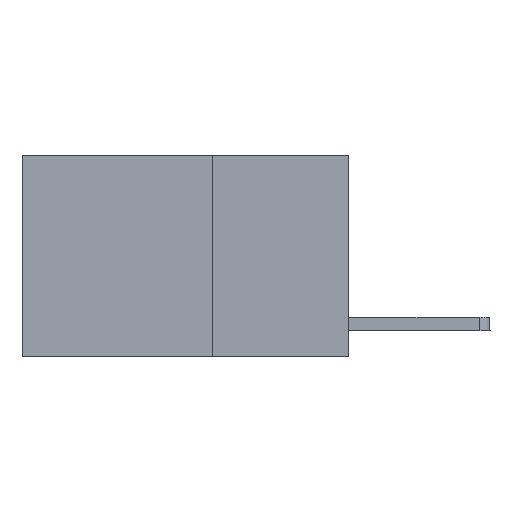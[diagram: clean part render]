
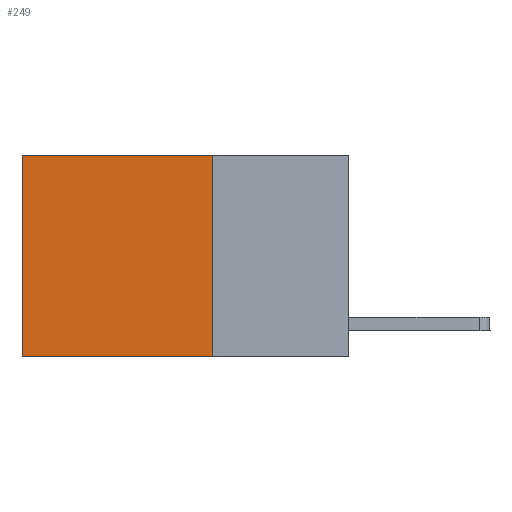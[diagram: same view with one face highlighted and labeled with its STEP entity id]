
A CAD part, left-side view. The second image highlights one B-rep face of the part: STEP entity #249.
In plain terms, the highlighted planar face has unit normal (-1, 0, 0).
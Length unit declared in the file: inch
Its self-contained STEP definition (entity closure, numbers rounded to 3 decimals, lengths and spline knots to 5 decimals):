
#249 = ADVANCED_FACE ( 'NONE', ( #1845 ), #5765, .F. ) ;
#305 = EDGE_CURVE ( 'NONE', #8486, #8757, #1118, .T. ) ;
#349 = ORIENTED_EDGE ( 'NONE', *, *, #305, .T. ) ;
#411 = LINE ( 'NONE', #3194, #6220 ) ;
#432 = EDGE_CURVE ( 'NONE', #8757, #2724, #976, .T. ) ;
#976 = LINE ( 'NONE', #3034, #7132 ) ;
#1118 = LINE ( 'NONE', #3878, #6696 ) ;
#1363 = LINE ( 'NONE', #4115, #3870 ) ;
#1447 = ORIENTED_EDGE ( 'NONE', *, *, #4941, .F. ) ;
#1714 = DIRECTION ( 'NONE',  ( 1., 0., 0. ) ) ;
#1845 = FACE_OUTER_BOUND ( 'NONE', #4244, .T. ) ;
#2724 = VERTEX_POINT ( 'NONE', #8836 ) ;
#2896 = CARTESIAN_POINT ( 'NONE',  ( 0.2625, 0.25, 0. ) ) ;
#3034 = CARTESIAN_POINT ( 'NONE',  ( 0.2625, 0.6, 0. ) ) ;
#3126 = DIRECTION ( 'NONE',  ( 0., 0., -1. ) ) ;
#3136 = CARTESIAN_POINT ( 'NONE',  ( 0.2625, 0.25, 0. ) ) ;
#3194 = CARTESIAN_POINT ( 'NONE',  ( 0.2625, 0.25, 0. ) ) ;
#3870 = VECTOR ( 'NONE', #7304, 39.37008 ) ;
#3878 = CARTESIAN_POINT ( 'NONE',  ( 0.2625, 0.25, 0. ) ) ;
#4075 = ORIENTED_EDGE ( 'NONE', *, *, #7503, .F. ) ;
#4115 = CARTESIAN_POINT ( 'NONE',  ( 0.2625, 0.25, -0.37 ) ) ;
#4244 = EDGE_LOOP ( 'NONE', ( #7293, #1447, #4075, #349 ) ) ;
#4474 = DIRECTION ( 'NONE',  ( 0., 0., -1. ) ) ;
#4941 = EDGE_CURVE ( 'NONE', #7408, #2724, #1363, .T. ) ;
#5765 = PLANE ( 'NONE',  #8844 ) ;
#6220 = VECTOR ( 'NONE', #8668, 39.37008 ) ;
#6623 = DIRECTION ( 'NONE',  ( 0., 1., 0. ) ) ;
#6696 = VECTOR ( 'NONE', #6623, 39.37008 ) ;
#7132 = VECTOR ( 'NONE', #3126, 39.37008 ) ;
#7293 = ORIENTED_EDGE ( 'NONE', *, *, #432, .T. ) ;
#7304 = DIRECTION ( 'NONE',  ( 0., 1., 0. ) ) ;
#7408 = VERTEX_POINT ( 'NONE', #7956 ) ;
#7503 = EDGE_CURVE ( 'NONE', #8486, #7408, #411, .T. ) ;
#7956 = CARTESIAN_POINT ( 'NONE',  ( 0.2625, 0.25, -0.37 ) ) ;
#8486 = VERTEX_POINT ( 'NONE', #2896 ) ;
#8668 = DIRECTION ( 'NONE',  ( 0., 0., -1. ) ) ;
#8757 = VERTEX_POINT ( 'NONE', #8934 ) ;
#8836 = CARTESIAN_POINT ( 'NONE',  ( 0.2625, 0.6, -0.37 ) ) ;
#8844 = AXIS2_PLACEMENT_3D ( 'NONE', #3136, #1714, #4474 ) ;
#8934 = CARTESIAN_POINT ( 'NONE',  ( 0.2625, 0.6, 0. ) ) ;
